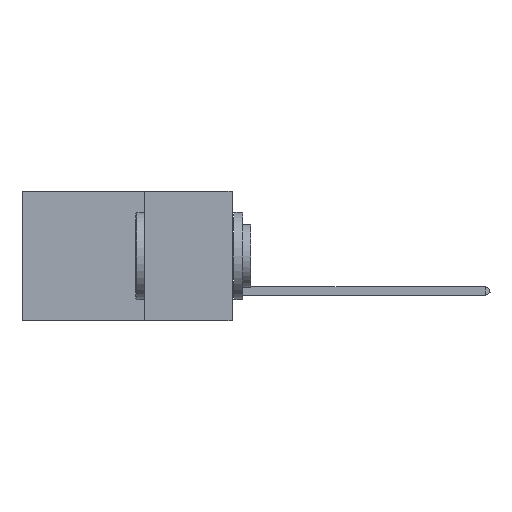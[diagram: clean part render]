
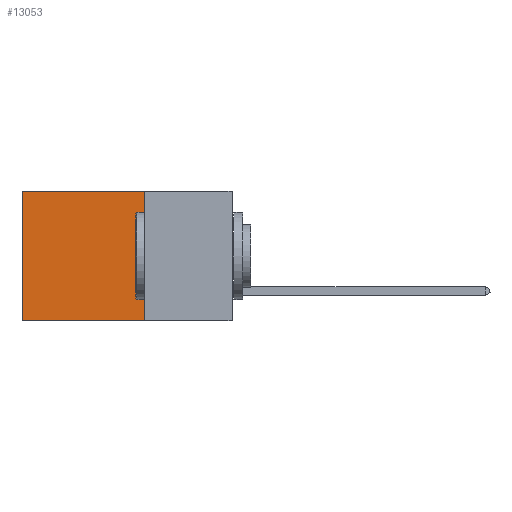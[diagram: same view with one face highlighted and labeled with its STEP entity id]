
A CAD part, left-side view. The second image highlights one B-rep face of the part: STEP entity #13053.
In plain terms, the highlighted planar face has unit normal (-1, 0, 0).
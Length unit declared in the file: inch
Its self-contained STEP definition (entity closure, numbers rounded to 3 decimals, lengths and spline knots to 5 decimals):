
#16 = CARTESIAN_POINT ( 'NONE',  ( 0.2875, 0.25, -0.37 ) ) ;
#252 = DIRECTION ( 'NONE',  ( 0., 0., -1. ) ) ;
#253 = CARTESIAN_POINT ( 'NONE',  ( 0.2875, 0.6, -0.37 ) ) ;
#286 = ORIENTED_EDGE ( 'NONE', *, *, #13304, .F. ) ;
#782 = VERTEX_POINT ( 'NONE', #7915 ) ;
#988 = ORIENTED_EDGE ( 'NONE', *, *, #4601, .T. ) ;
#1830 = CARTESIAN_POINT ( 'NONE',  ( 0.2875, 0.25, 0. ) ) ;
#2230 = CARTESIAN_POINT ( 'NONE',  ( 0.2875, 0.25, 0. ) ) ;
#2428 = CARTESIAN_POINT ( 'NONE',  ( 0.2875, 0.6, 0. ) ) ;
#3924 = VECTOR ( 'NONE', #6667, 39.37008 ) ;
#4049 = AXIS2_PLACEMENT_3D ( 'NONE', #4641, #6796, #7878 ) ;
#4164 = LINE ( 'NONE', #2428, #12302 ) ;
#4214 = EDGE_CURVE ( 'NONE', #7945, #10904, #4164, .T. ) ;
#4548 = VERTEX_POINT ( 'NONE', #11699 ) ;
#4601 = EDGE_CURVE ( 'NONE', #4548, #7945, #7995, .T. ) ;
#4641 = CARTESIAN_POINT ( 'NONE',  ( 0.2875, 0.25, 0. ) ) ;
#6263 = VECTOR ( 'NONE', #7619, 39.37008 ) ;
#6667 = DIRECTION ( 'NONE',  ( 0., 0., -1. ) ) ;
#6796 = DIRECTION ( 'NONE',  ( 1., 0., 0. ) ) ;
#7619 = DIRECTION ( 'NONE',  ( 0., 1., 0. ) ) ;
#7878 = DIRECTION ( 'NONE',  ( 0., 0., -1. ) ) ;
#7915 = CARTESIAN_POINT ( 'NONE',  ( 0.2875, 0.25, -0.37 ) ) ;
#7945 = VERTEX_POINT ( 'NONE', #13265 ) ;
#7995 = LINE ( 'NONE', #1830, #10221 ) ;
#8316 = EDGE_LOOP ( 'NONE', ( #10353, #12380, #286, #988 ) ) ;
#8647 = FACE_OUTER_BOUND ( 'NONE', #8316, .T. ) ;
#8845 = PLANE ( 'NONE',  #4049 ) ;
#9388 = DIRECTION ( 'NONE',  ( 0., 1., 0. ) ) ;
#9829 = LINE ( 'NONE', #2230, #3924 ) ;
#10221 = VECTOR ( 'NONE', #9388, 39.37008 ) ;
#10353 = ORIENTED_EDGE ( 'NONE', *, *, #4214, .T. ) ;
#10859 = LINE ( 'NONE', #16, #6263 ) ;
#10904 = VERTEX_POINT ( 'NONE', #253 ) ;
#11699 = CARTESIAN_POINT ( 'NONE',  ( 0.2875, 0.25, 0. ) ) ;
#12302 = VECTOR ( 'NONE', #252, 39.37008 ) ;
#12380 = ORIENTED_EDGE ( 'NONE', *, *, #13578, .F. ) ;
#13053 = ADVANCED_FACE ( 'NONE', ( #8647 ), #8845, .F. ) ;
#13265 = CARTESIAN_POINT ( 'NONE',  ( 0.2875, 0.6, 0. ) ) ;
#13304 = EDGE_CURVE ( 'NONE', #4548, #782, #9829, .T. ) ;
#13578 = EDGE_CURVE ( 'NONE', #782, #10904, #10859, .T. ) ;
